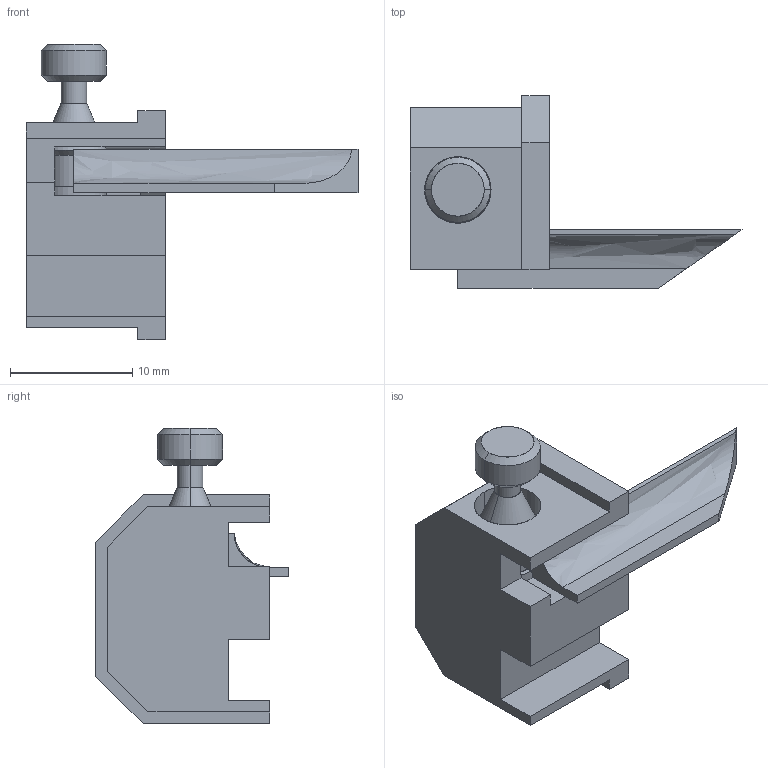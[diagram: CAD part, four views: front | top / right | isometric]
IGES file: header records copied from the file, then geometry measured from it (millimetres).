
Start section: SolidWorks IGES file using analytic representation for surfaces
Global section: file name: Auto Sear Assy.IGS; native system: SolidWorks 2012; preprocessor: SolidWorks 2012; author: W.Morrison; date: 120906.063031; units: inch
Bounding box: 27.16 x 15.75 x 24.16 mm (x, y, z)
Surface area: 2433.4 mm2 (no closed solid volume)
Topology: 0 solids, 0 shells, 82 faces, 928 edges, 928 vertices
Faces by surface type: bspline 53, revolution 29
